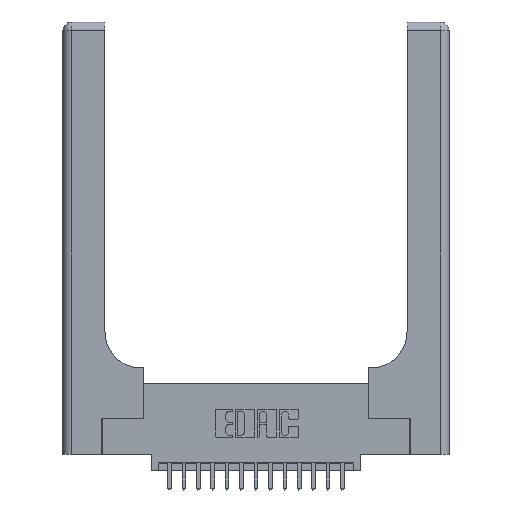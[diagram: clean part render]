
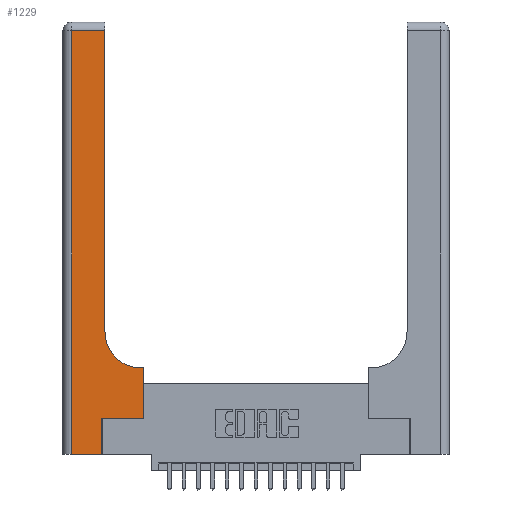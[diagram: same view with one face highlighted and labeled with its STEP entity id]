
A CAD part, top view. The second image highlights one B-rep face of the part: STEP entity #1229.
In plain terms, the highlighted planar face has unit normal (0, 0, 1).
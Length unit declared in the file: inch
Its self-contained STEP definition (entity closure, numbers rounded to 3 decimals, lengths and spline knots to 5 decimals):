
#48 = ORIENTED_EDGE ( 'NONE', *, *, #14917, .T. ) ;
#182 = LINE ( 'NONE', #18875, #4184 ) ;
#1229 = ADVANCED_FACE ( 'NONE', ( #13647 ), #15926, .F. ) ;
#1247 = VECTOR ( 'NONE', #6822, 39.37008 ) ;
#1299 = AXIS2_PLACEMENT_3D ( 'NONE', #13294, #7021, #16056 ) ;
#1764 = CARTESIAN_POINT ( 'NONE',  ( 0.5585, 0.6, 0.37 ) ) ;
#2058 = DIRECTION ( 'NONE',  ( 0., -1., 0. ) ) ;
#2121 = CARTESIAN_POINT ( 'NONE',  ( 0.06, 3., 0.37 ) ) ;
#2219 = VECTOR ( 'NONE', #16134, 39.37008 ) ;
#2584 = EDGE_CURVE ( 'NONE', #4832, #14713, #5160, .T. ) ;
#2821 = EDGE_LOOP ( 'NONE', ( #8022, #11025, #18682, #18661, #5743, #6844, #48, #8210, #4906 ) ) ;
#3107 = DIRECTION ( 'NONE',  ( 1., 0., 0. ) ) ;
#3136 = EDGE_CURVE ( 'NONE', #14280, #15685, #17108, .T. ) ;
#3817 = CARTESIAN_POINT ( 'NONE',  ( 0.269, 0., 0.37 ) ) ;
#4184 = VECTOR ( 'NONE', #5478, 39.37008 ) ;
#4802 = LINE ( 'NONE', #2121, #11830 ) ;
#4832 = VERTEX_POINT ( 'NONE', #15174 ) ;
#4906 = ORIENTED_EDGE ( 'NONE', *, *, #16731, .T. ) ;
#5160 = LINE ( 'NONE', #16140, #12889 ) ;
#5385 = CARTESIAN_POINT ( 'NONE',  ( 0.5415, 0.6, 0.37 ) ) ;
#5478 = DIRECTION ( 'NONE',  ( -1., 0., 0. ) ) ;
#5743 = ORIENTED_EDGE ( 'NONE', *, *, #3136, .T. ) ;
#5914 = CARTESIAN_POINT ( 'NONE',  ( 0., 2.94, 0.37 ) ) ;
#6071 = CIRCLE ( 'NONE', #1299, 0.25 ) ;
#6347 = DIRECTION ( 'NONE',  ( 1., 0., 0. ) ) ;
#6473 = CARTESIAN_POINT ( 'NONE',  ( 0.06, 0., 0.37 ) ) ;
#6803 = VERTEX_POINT ( 'NONE', #6473 ) ;
#6822 = DIRECTION ( 'NONE',  ( 0., 1., 0. ) ) ;
#6844 = ORIENTED_EDGE ( 'NONE', *, *, #13566, .T. ) ;
#7021 = DIRECTION ( 'NONE',  ( 0., 0., -1. ) ) ;
#7205 = VERTEX_POINT ( 'NONE', #12747 ) ;
#8022 = ORIENTED_EDGE ( 'NONE', *, *, #2584, .T. ) ;
#8210 = ORIENTED_EDGE ( 'NONE', *, *, #11710, .T. ) ;
#9074 = VERTEX_POINT ( 'NONE', #1764 ) ;
#9159 = CARTESIAN_POINT ( 'NONE',  ( 0.06, 2.94, 0.37 ) ) ;
#9182 = LINE ( 'NONE', #13704, #11538 ) ;
#9488 = LINE ( 'NONE', #5914, #2219 ) ;
#9737 = VECTOR ( 'NONE', #6347, 39.37008 ) ;
#9988 = DIRECTION ( 'NONE',  ( 0., 1., 0. ) ) ;
#10730 = AXIS2_PLACEMENT_3D ( 'NONE', #17537, #11422, #18774 ) ;
#11025 = ORIENTED_EDGE ( 'NONE', *, *, #17903, .T. ) ;
#11087 = CARTESIAN_POINT ( 'NONE',  ( 0.2915, 2.94, 0.37 ) ) ;
#11422 = DIRECTION ( 'NONE',  ( 0., 0., -1. ) ) ;
#11538 = VECTOR ( 'NONE', #3107, 39.37008 ) ;
#11702 = CARTESIAN_POINT ( 'NONE',  ( 0.269, 0., 0.37 ) ) ;
#11710 = EDGE_CURVE ( 'NONE', #9074, #17728, #182, .T. ) ;
#11782 = CARTESIAN_POINT ( 'NONE',  ( 0.269, 0.25, 0.37 ) ) ;
#11830 = VECTOR ( 'NONE', #2058, 39.37008 ) ;
#12053 = LINE ( 'NONE', #12968, #1247 ) ;
#12747 = CARTESIAN_POINT ( 'NONE',  ( 0.5585, 0.25, 0.37 ) ) ;
#12889 = VECTOR ( 'NONE', #9988, 39.37008 ) ;
#12968 = CARTESIAN_POINT ( 'NONE',  ( 0.5585, 0.25, 0.37 ) ) ;
#13294 = CARTESIAN_POINT ( 'NONE',  ( 0.5415, 0.85, 0.37 ) ) ;
#13499 = VERTEX_POINT ( 'NONE', #9159 ) ;
#13566 = EDGE_CURVE ( 'NONE', #15685, #7205, #17958, .T. ) ;
#13647 = FACE_OUTER_BOUND ( 'NONE', #2821, .T. ) ;
#13704 = CARTESIAN_POINT ( 'NONE',  ( 0., 0., 0.37 ) ) ;
#13762 = EDGE_CURVE ( 'NONE', #13499, #6803, #4802, .T. ) ;
#14280 = VERTEX_POINT ( 'NONE', #11702 ) ;
#14713 = VERTEX_POINT ( 'NONE', #11087 ) ;
#14917 = EDGE_CURVE ( 'NONE', #7205, #9074, #12053, .T. ) ;
#15174 = CARTESIAN_POINT ( 'NONE',  ( 0.2915, 0.85, 0.37 ) ) ;
#15231 = CARTESIAN_POINT ( 'NONE',  ( 0.269, 0.25, 0.37 ) ) ;
#15685 = VERTEX_POINT ( 'NONE', #11782 ) ;
#15912 = DIRECTION ( 'NONE',  ( 0., 1., 0. ) ) ;
#15926 = PLANE ( 'NONE',  #10730 ) ;
#16056 = DIRECTION ( 'NONE',  ( 1., 0., 0. ) ) ;
#16134 = DIRECTION ( 'NONE',  ( -1., 0., 0. ) ) ;
#16140 = CARTESIAN_POINT ( 'NONE',  ( 0.2915, 3., 0.37 ) ) ;
#16149 = VECTOR ( 'NONE', #15912, 39.37008 ) ;
#16333 = EDGE_CURVE ( 'NONE', #6803, #14280, #9182, .T. ) ;
#16731 = EDGE_CURVE ( 'NONE', #17728, #4832, #6071, .T. ) ;
#17108 = LINE ( 'NONE', #3817, #16149 ) ;
#17537 = CARTESIAN_POINT ( 'NONE',  ( 0., 3., 0.37 ) ) ;
#17728 = VERTEX_POINT ( 'NONE', #5385 ) ;
#17903 = EDGE_CURVE ( 'NONE', #14713, #13499, #9488, .T. ) ;
#17958 = LINE ( 'NONE', #15231, #9737 ) ;
#18661 = ORIENTED_EDGE ( 'NONE', *, *, #16333, .T. ) ;
#18682 = ORIENTED_EDGE ( 'NONE', *, *, #13762, .T. ) ;
#18774 = DIRECTION ( 'NONE',  ( -1., 0., 0. ) ) ;
#18875 = CARTESIAN_POINT ( 'NONE',  ( 0.2915, 0.6, 0.37 ) ) ;
